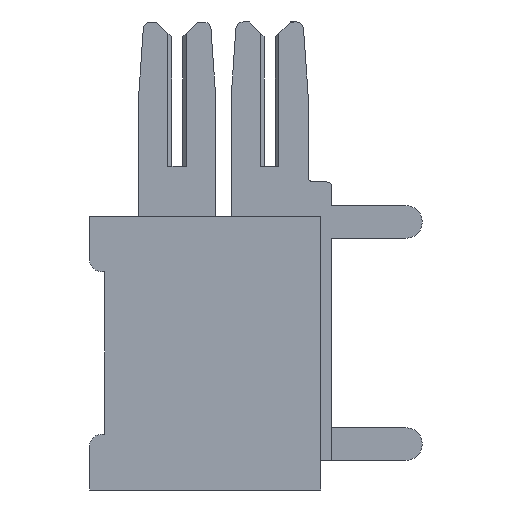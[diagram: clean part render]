
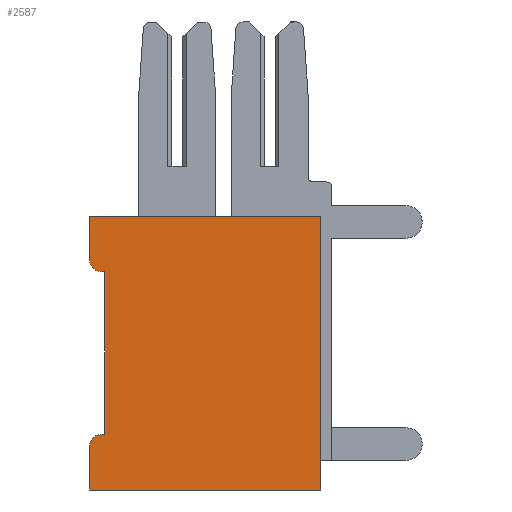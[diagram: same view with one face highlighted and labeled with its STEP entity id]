
A CAD part, left-side view. The second image highlights one B-rep face of the part: STEP entity #2587.
In plain terms, the highlighted planar face has unit normal (-1, 0, 0).
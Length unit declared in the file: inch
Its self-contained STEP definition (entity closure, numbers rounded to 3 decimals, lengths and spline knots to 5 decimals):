
#149 = LINE ( 'NONE', #3635, #1381 ) ;
#201 = VERTEX_POINT ( 'NONE', #3367 ) ;
#229 = CARTESIAN_POINT ( 'NONE',  ( 0., 0., -0.37 ) ) ;
#408 = CARTESIAN_POINT ( 'NONE',  ( 0., 0., -0.37 ) ) ;
#479 = ORIENTED_EDGE ( 'NONE', *, *, #2082, .T. ) ;
#501 = EDGE_CURVE ( 'NONE', #1703, #2037, #149, .T. ) ;
#504 = DIRECTION ( 'NONE',  ( 0., -1., 0. ) ) ;
#510 = DIRECTION ( 'NONE',  ( 0., 0., 1. ) ) ;
#540 = VERTEX_POINT ( 'NONE', #4147 ) ;
#547 = LINE ( 'NONE', #3317, #6982 ) ;
#740 = ORIENTED_EDGE ( 'NONE', *, *, #4113, .F. ) ;
#750 = DIRECTION ( 'NONE',  ( 0., -1., 0. ) ) ;
#802 = ORIENTED_EDGE ( 'NONE', *, *, #2321, .F. ) ;
#1024 = CARTESIAN_POINT ( 'NONE',  ( 0., 0.312, -0.075 ) ) ;
#1084 = DIRECTION ( 'NONE',  ( 0., 0., 1. ) ) ;
#1179 = VERTEX_POINT ( 'NONE', #3184 ) ;
#1285 = EDGE_CURVE ( 'NONE', #3556, #540, #6237, .T. ) ;
#1381 = VECTOR ( 'NONE', #5828, 39.37008 ) ;
#1407 = DIRECTION ( 'NONE',  ( 0., -1., 0. ) ) ;
#1551 = VERTEX_POINT ( 'NONE', #4474 ) ;
#1703 = VERTEX_POINT ( 'NONE', #4945 ) ;
#1724 = EDGE_CURVE ( 'NONE', #4902, #1551, #6835, .T. ) ;
#1845 = DIRECTION ( 'NONE',  ( 0., 0., 1. ) ) ;
#1874 = CARTESIAN_POINT ( 'NONE',  ( 0., 0.297, -0.31 ) ) ;
#2018 = CARTESIAN_POINT ( 'NONE',  ( 0., 0.312, -0.295 ) ) ;
#2037 = VERTEX_POINT ( 'NONE', #3576 ) ;
#2076 = CARTESIAN_POINT ( 'NONE',  ( 0., 0.292, -0.075 ) ) ;
#2082 = EDGE_CURVE ( 'NONE', #1179, #3463, #2221, .T. ) ;
#2218 = CARTESIAN_POINT ( 'NONE',  ( 0., 0.312, -0.31 ) ) ;
#2221 = CIRCLE ( 'NONE', #3897, 0.015 ) ;
#2245 = CARTESIAN_POINT ( 'NONE',  ( 0., 0.292, -0.295 ) ) ;
#2321 = EDGE_CURVE ( 'NONE', #1179, #6363, #6649, .T. ) ;
#2476 = LINE ( 'NONE', #2245, #5700 ) ;
#2587 = ADVANCED_FACE ( 'NONE', ( #3878 ), #2718, .T. ) ;
#2662 = CARTESIAN_POINT ( 'NONE',  ( 0., 0.292, -0.295 ) ) ;
#2718 = PLANE ( 'NONE',  #3527 ) ;
#2889 = EDGE_CURVE ( 'NONE', #201, #3556, #3542, .T. ) ;
#3031 = EDGE_LOOP ( 'NONE', ( #5235, #4930, #3089, #5790, #802, #479, #740, #3816, #4874, #6885 ) ) ;
#3089 = ORIENTED_EDGE ( 'NONE', *, *, #1724, .F. ) ;
#3184 = CARTESIAN_POINT ( 'NONE',  ( 0., 0.297, -0.295 ) ) ;
#3268 = DIRECTION ( 'NONE',  ( 0., 0., 1. ) ) ;
#3283 = EDGE_CURVE ( 'NONE', #2037, #540, #4487, .T. ) ;
#3317 = CARTESIAN_POINT ( 'NONE',  ( 0., 0.312, -0.37 ) ) ;
#3367 = CARTESIAN_POINT ( 'NONE',  ( 0., 0.312, -0.37 ) ) ;
#3463 = VERTEX_POINT ( 'NONE', #2218 ) ;
#3479 = CARTESIAN_POINT ( 'NONE',  ( 0., 0.297, -0.06 ) ) ;
#3527 = AXIS2_PLACEMENT_3D ( 'NONE', #6084, #4424, #1084 ) ;
#3542 = LINE ( 'NONE', #229, #3791 ) ;
#3556 = VERTEX_POINT ( 'NONE', #4594 ) ;
#3569 = EDGE_CURVE ( 'NONE', #1703, #1551, #4559, .T. ) ;
#3576 = CARTESIAN_POINT ( 'NONE',  ( 0., 0.312, 0. ) ) ;
#3635 = CARTESIAN_POINT ( 'NONE',  ( 0., 0.312, -0.37 ) ) ;
#3791 = VECTOR ( 'NONE', #750, 39.37008 ) ;
#3816 = ORIENTED_EDGE ( 'NONE', *, *, #2889, .T. ) ;
#3860 = CARTESIAN_POINT ( 'NONE',  ( 0., 0., 0. ) ) ;
#3863 = DIRECTION ( 'NONE',  ( 0., 1., 0. ) ) ;
#3878 = FACE_OUTER_BOUND ( 'NONE', #3031, .T. ) ;
#3897 = AXIS2_PLACEMENT_3D ( 'NONE', #1874, #6415, #6368 ) ;
#4113 = EDGE_CURVE ( 'NONE', #201, #3463, #547, .T. ) ;
#4147 = CARTESIAN_POINT ( 'NONE',  ( 0., 0., 0. ) ) ;
#4311 = VECTOR ( 'NONE', #1407, 39.37008 ) ;
#4424 = DIRECTION ( 'NONE',  ( -1., 0., 0. ) ) ;
#4474 = CARTESIAN_POINT ( 'NONE',  ( 0., 0.297, -0.075 ) ) ;
#4487 = LINE ( 'NONE', #3860, #7172 ) ;
#4559 = CIRCLE ( 'NONE', #4609, 0.015 ) ;
#4594 = CARTESIAN_POINT ( 'NONE',  ( 0., 0., -0.37 ) ) ;
#4609 = AXIS2_PLACEMENT_3D ( 'NONE', #3479, #5741, #1845 ) ;
#4830 = EDGE_CURVE ( 'NONE', #6363, #4902, #2476, .T. ) ;
#4874 = ORIENTED_EDGE ( 'NONE', *, *, #1285, .T. ) ;
#4902 = VERTEX_POINT ( 'NONE', #2076 ) ;
#4930 = ORIENTED_EDGE ( 'NONE', *, *, #3569, .T. ) ;
#4945 = CARTESIAN_POINT ( 'NONE',  ( 0., 0.312, -0.06 ) ) ;
#5019 = VECTOR ( 'NONE', #3863, 39.37008 ) ;
#5235 = ORIENTED_EDGE ( 'NONE', *, *, #501, .F. ) ;
#5700 = VECTOR ( 'NONE', #510, 39.37008 ) ;
#5741 = DIRECTION ( 'NONE',  ( -1., 0., 0. ) ) ;
#5790 = ORIENTED_EDGE ( 'NONE', *, *, #4830, .F. ) ;
#5828 = DIRECTION ( 'NONE',  ( 0., 0., 1. ) ) ;
#6084 = CARTESIAN_POINT ( 'NONE',  ( 0., 0., -0.37 ) ) ;
#6098 = DIRECTION ( 'NONE',  ( 0., 0., 1. ) ) ;
#6237 = LINE ( 'NONE', #408, #6841 ) ;
#6363 = VERTEX_POINT ( 'NONE', #2662 ) ;
#6368 = DIRECTION ( 'NONE',  ( 0., 0., 1. ) ) ;
#6415 = DIRECTION ( 'NONE',  ( -1., 0., 0. ) ) ;
#6649 = LINE ( 'NONE', #2018, #4311 ) ;
#6835 = LINE ( 'NONE', #1024, #5019 ) ;
#6841 = VECTOR ( 'NONE', #6098, 39.37008 ) ;
#6885 = ORIENTED_EDGE ( 'NONE', *, *, #3283, .F. ) ;
#6982 = VECTOR ( 'NONE', #3268, 39.37008 ) ;
#7172 = VECTOR ( 'NONE', #504, 39.37008 ) ;
